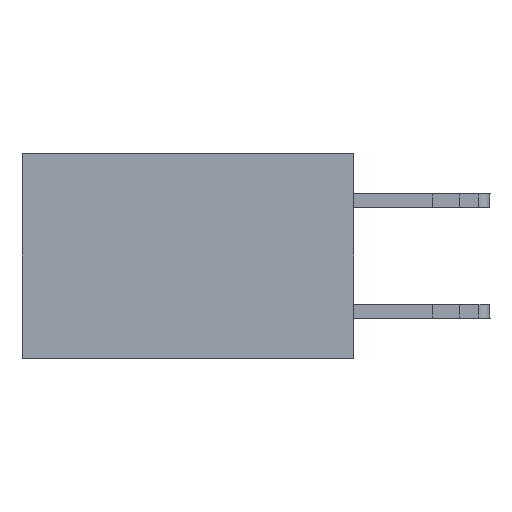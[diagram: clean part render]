
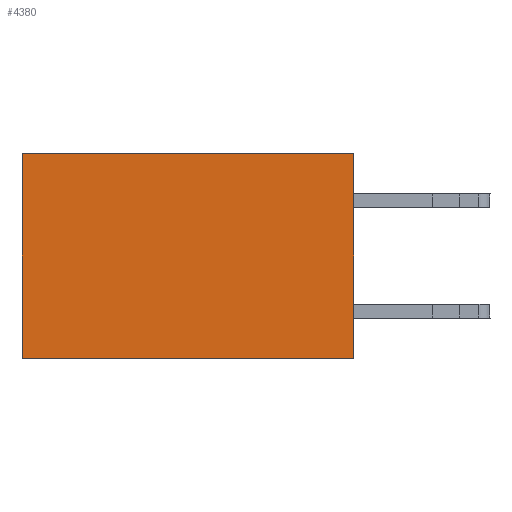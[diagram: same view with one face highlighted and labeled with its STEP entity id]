
A CAD part, left-side view. The second image highlights one B-rep face of the part: STEP entity #4380.
In plain terms, the highlighted planar face has unit normal (-1, 0, 0).
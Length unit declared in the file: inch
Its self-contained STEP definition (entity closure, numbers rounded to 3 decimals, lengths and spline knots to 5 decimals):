
#1074 = EDGE_CURVE ( 'NONE', #9735, #33250, #29553, .T. ) ;
#2166 = DIRECTION ( 'NONE',  ( 0., 1., 0. ) ) ;
#3165 = DIRECTION ( 'NONE',  ( 1., 0., 0. ) ) ;
#4380 = ADVANCED_FACE ( 'NONE', ( #21484 ), #31448, .F. ) ;
#4746 = EDGE_LOOP ( 'NONE', ( #25780, #17050, #14214, #30686 ) ) ;
#5338 = EDGE_CURVE ( 'NONE', #9735, #15672, #30501, .T. ) ;
#6347 = VECTOR ( 'NONE', #2166, 39.37008 ) ;
#8138 = VECTOR ( 'NONE', #32713, 39.37008 ) ;
#9364 = CARTESIAN_POINT ( 'NONE',  ( 0.2875, 0., 0. ) ) ;
#9735 = VERTEX_POINT ( 'NONE', #16064 ) ;
#9888 = DIRECTION ( 'NONE',  ( 0., 0., -1. ) ) ;
#14214 = ORIENTED_EDGE ( 'NONE', *, *, #1074, .F. ) ;
#15215 = EDGE_CURVE ( 'NONE', #15672, #36474, #23755, .T. ) ;
#15467 = CARTESIAN_POINT ( 'NONE',  ( 0.2875, 0.6, 0. ) ) ;
#15672 = VERTEX_POINT ( 'NONE', #15467 ) ;
#16064 = CARTESIAN_POINT ( 'NONE',  ( 0.2875, 0., 0. ) ) ;
#17050 = ORIENTED_EDGE ( 'NONE', *, *, #33107, .F. ) ;
#17936 = CARTESIAN_POINT ( 'NONE',  ( 0.2875, 0.6, -0.37 ) ) ;
#18947 = CARTESIAN_POINT ( 'NONE',  ( 0.2875, 0., 0. ) ) ;
#20502 = CARTESIAN_POINT ( 'NONE',  ( 0.2875, 0.6, 0. ) ) ;
#21085 = VECTOR ( 'NONE', #27448, 39.37008 ) ;
#21484 = FACE_OUTER_BOUND ( 'NONE', #4746, .T. ) ;
#23755 = LINE ( 'NONE', #20502, #35926 ) ;
#25186 = LINE ( 'NONE', #35816, #6347 ) ;
#25780 = ORIENTED_EDGE ( 'NONE', *, *, #15215, .T. ) ;
#27105 = CARTESIAN_POINT ( 'NONE',  ( 0.2875, 0., 0. ) ) ;
#27448 = DIRECTION ( 'NONE',  ( 0., 1., 0. ) ) ;
#29553 = LINE ( 'NONE', #27105, #8138 ) ;
#30501 = LINE ( 'NONE', #18947, #21085 ) ;
#30686 = ORIENTED_EDGE ( 'NONE', *, *, #5338, .T. ) ;
#31448 = PLANE ( 'NONE',  #33178 ) ;
#32029 = CARTESIAN_POINT ( 'NONE',  ( 0.2875, 0., -0.37 ) ) ;
#32713 = DIRECTION ( 'NONE',  ( 0., 0., -1. ) ) ;
#33107 = EDGE_CURVE ( 'NONE', #33250, #36474, #25186, .T. ) ;
#33178 = AXIS2_PLACEMENT_3D ( 'NONE', #9364, #3165, #34475 ) ;
#33250 = VERTEX_POINT ( 'NONE', #32029 ) ;
#34475 = DIRECTION ( 'NONE',  ( 0., 0., -1. ) ) ;
#35816 = CARTESIAN_POINT ( 'NONE',  ( 0.2875, 0., -0.37 ) ) ;
#35926 = VECTOR ( 'NONE', #9888, 39.37008 ) ;
#36474 = VERTEX_POINT ( 'NONE', #17936 ) ;
